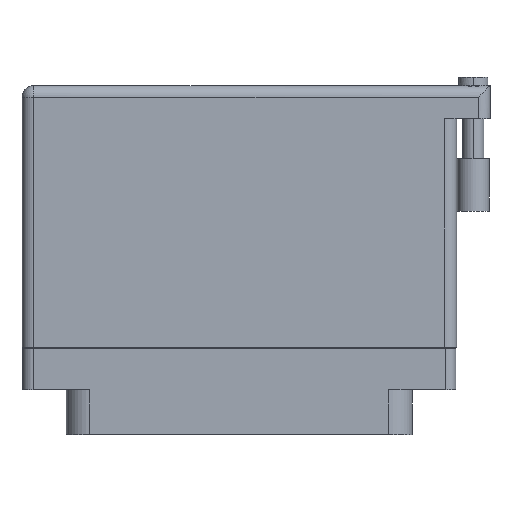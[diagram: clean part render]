
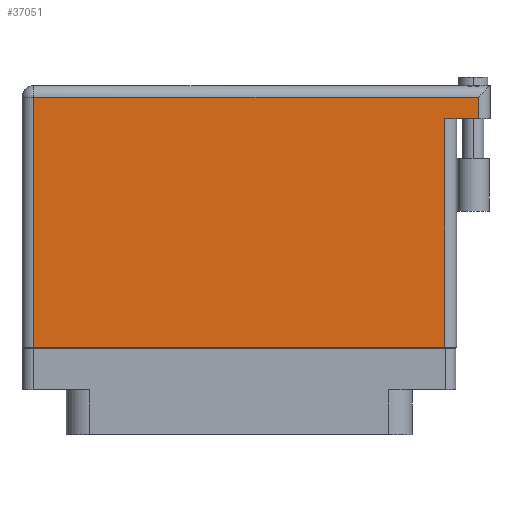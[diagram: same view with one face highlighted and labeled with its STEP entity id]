
A CAD part, front view. The second image highlights one B-rep face of the part: STEP entity #37051.
In plain terms, the highlighted face is planar.
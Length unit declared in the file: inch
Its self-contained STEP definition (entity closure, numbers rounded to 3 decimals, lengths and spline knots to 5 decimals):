
#715 = VECTOR ( 'NONE', #46669, 39.37008 ) ;
#1387 = VECTOR ( 'NONE', #33221, 39.37008 ) ;
#4666 = FACE_OUTER_BOUND ( 'NONE', #43550, .T. ) ;
#4676 = VECTOR ( 'NONE', #32967, 39.37008 ) ;
#7061 = ORIENTED_EDGE ( 'NONE', *, *, #46757, .F. ) ;
#7803 = LINE ( 'NONE', #25088, #4676 ) ;
#10302 = VERTEX_POINT ( 'NONE', #35007 ) ;
#10691 = EDGE_CURVE ( 'NONE', #15998, #42015, #34443, .T. ) ;
#12931 = CARTESIAN_POINT ( 'NONE',  ( -1.3, 1.466, 0.4495 ) ) ;
#13804 = CARTESIAN_POINT ( 'NONE',  ( 1.43, 1.269, 0.4495 ) ) ;
#15238 = CARTESIAN_POINT ( 'NONE',  ( -1.23, -0.1, 0.4495 ) ) ;
#15998 = VERTEX_POINT ( 'NONE', #38924 ) ;
#16366 = EDGE_CURVE ( 'NONE', #42015, #10302, #22885, .T. ) ;
#20115 = DIRECTION ( 'NONE',  ( -1., 0., 0. ) ) ;
#20546 = PLANE ( 'NONE',  #24362 ) ;
#20628 = LINE ( 'NONE', #15238, #715 ) ;
#22385 = CARTESIAN_POINT ( 'NONE',  ( 1.43, 1.396, 0.4495 ) ) ;
#22731 = CARTESIAN_POINT ( 'NONE',  ( -1.23, 1.396, 0.4495 ) ) ;
#22885 = LINE ( 'NONE', #41712, #40383 ) ;
#23467 = CARTESIAN_POINT ( 'NONE',  ( -1.3, -0.1, 0.4495 ) ) ;
#24272 = VECTOR ( 'NONE', #20115, 39.37008 ) ;
#24362 = AXIS2_PLACEMENT_3D ( 'NONE', #12931, #40807, #48206 ) ;
#25088 = CARTESIAN_POINT ( 'NONE',  ( -1.3, 1.396, 0.4495 ) ) ;
#27352 = ORIENTED_EDGE ( 'NONE', *, *, #33157, .T. ) ;
#29598 = DIRECTION ( 'NONE',  ( 0., 1., 0. ) ) ;
#31435 = EDGE_CURVE ( 'NONE', #34313, #49766, #42533, .T. ) ;
#31821 = VECTOR ( 'NONE', #45533, 39.37008 ) ;
#32967 = DIRECTION ( 'NONE',  ( -1., 0., 0. ) ) ;
#33157 = EDGE_CURVE ( 'NONE', #35584, #15998, #20628, .T. ) ;
#33221 = DIRECTION ( 'NONE',  ( 1., 0., 0. ) ) ;
#33406 = ORIENTED_EDGE ( 'NONE', *, *, #10691, .T. ) ;
#34313 = VERTEX_POINT ( 'NONE', #13804 ) ;
#34443 = LINE ( 'NONE', #23467, #1387 ) ;
#35007 = CARTESIAN_POINT ( 'NONE',  ( 1.23, 1.269, 0.4495 ) ) ;
#35584 = VERTEX_POINT ( 'NONE', #22731 ) ;
#37051 = ADVANCED_FACE ( 'NONE', ( #4666 ), #20546, .F. ) ;
#38924 = CARTESIAN_POINT ( 'NONE',  ( -1.23, -0.1, 0.4495 ) ) ;
#39108 = CARTESIAN_POINT ( 'NONE',  ( 1.23, -0.1, 0.4495 ) ) ;
#40383 = VECTOR ( 'NONE', #29598, 39.37008 ) ;
#40807 = DIRECTION ( 'NONE',  ( 0., 0., -1. ) ) ;
#41480 = CARTESIAN_POINT ( 'NONE',  ( 1.43, 1.466, 0.4495 ) ) ;
#41712 = CARTESIAN_POINT ( 'NONE',  ( 1.23, 1.269, 0.4495 ) ) ;
#42015 = VERTEX_POINT ( 'NONE', #39108 ) ;
#42533 = LINE ( 'NONE', #41480, #31821 ) ;
#43003 = EDGE_CURVE ( 'NONE', #49766, #35584, #7803, .T. ) ;
#43550 = EDGE_LOOP ( 'NONE', ( #33406, #45388, #7061, #46170, #50622, #27352 ) ) ;
#44084 = CARTESIAN_POINT ( 'NONE',  ( 1.5, 1.269, 0.4495 ) ) ;
#45388 = ORIENTED_EDGE ( 'NONE', *, *, #16366, .T. ) ;
#45533 = DIRECTION ( 'NONE',  ( 0., 1., 0. ) ) ;
#45618 = LINE ( 'NONE', #44084, #24272 ) ;
#46170 = ORIENTED_EDGE ( 'NONE', *, *, #31435, .T. ) ;
#46669 = DIRECTION ( 'NONE',  ( 0., -1., 0. ) ) ;
#46757 = EDGE_CURVE ( 'NONE', #34313, #10302, #45618, .T. ) ;
#48206 = DIRECTION ( 'NONE',  ( -1., 0., 0. ) ) ;
#49766 = VERTEX_POINT ( 'NONE', #22385 ) ;
#50622 = ORIENTED_EDGE ( 'NONE', *, *, #43003, .T. ) ;
